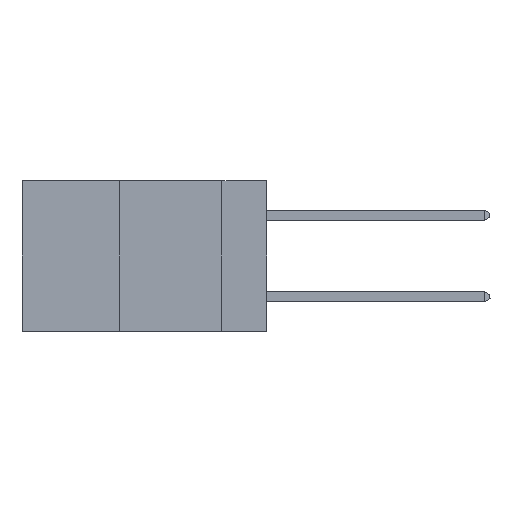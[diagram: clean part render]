
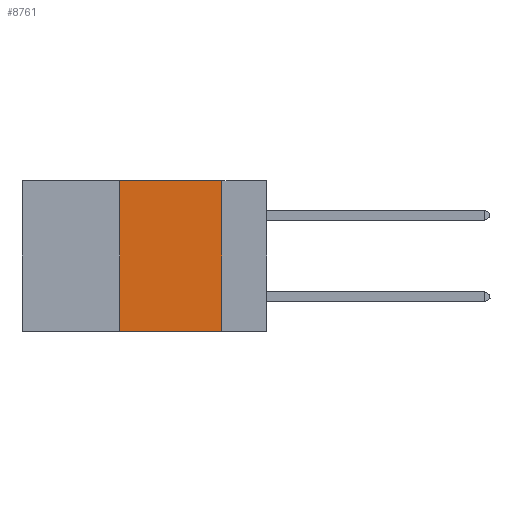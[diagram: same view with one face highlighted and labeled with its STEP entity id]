
A CAD part, left-side view. The second image highlights one B-rep face of the part: STEP entity #8761.
In plain terms, the highlighted planar face has unit normal (-1, 0, 0).
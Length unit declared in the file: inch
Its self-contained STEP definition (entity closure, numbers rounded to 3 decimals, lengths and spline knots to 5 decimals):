
#80 = LINE ( 'NONE', #5714, #9266 ) ;
#611 = DIRECTION ( 'NONE',  ( 0., 0., 1. ) ) ;
#1285 = EDGE_CURVE ( 'NONE', #9797, #2730, #80, .T. ) ;
#1292 = EDGE_CURVE ( 'NONE', #9797, #6318, #3697, .T. ) ;
#1509 = DIRECTION ( 'NONE',  ( 1., 0., 0. ) ) ;
#1845 = ORIENTED_EDGE ( 'NONE', *, *, #2456, .F. ) ;
#1931 = CARTESIAN_POINT ( 'NONE',  ( 0., 0.11, -0.37 ) ) ;
#2225 = FACE_OUTER_BOUND ( 'NONE', #6689, .T. ) ;
#2456 = EDGE_CURVE ( 'NONE', #7040, #6318, #9133, .T. ) ;
#2730 = VERTEX_POINT ( 'NONE', #5146 ) ;
#3697 = LINE ( 'NONE', #6640, #4223 ) ;
#3983 = PLANE ( 'NONE',  #10372 ) ;
#4223 = VECTOR ( 'NONE', #7470, 39.37008 ) ;
#4244 = DIRECTION ( 'NONE',  ( 0., -1., 0. ) ) ;
#4284 = CARTESIAN_POINT ( 'NONE',  ( 0., 0.6, 0. ) ) ;
#4816 = ORIENTED_EDGE ( 'NONE', *, *, #8302, .F. ) ;
#5146 = CARTESIAN_POINT ( 'NONE',  ( 0., 0.36, 0. ) ) ;
#5529 = ORIENTED_EDGE ( 'NONE', *, *, #1292, .T. ) ;
#5714 = CARTESIAN_POINT ( 'NONE',  ( 0., 0.36, 0. ) ) ;
#5935 = DIRECTION ( 'NONE',  ( 0., 0., -1. ) ) ;
#6318 = VERTEX_POINT ( 'NONE', #1931 ) ;
#6640 = CARTESIAN_POINT ( 'NONE',  ( 0., 0.6, -0.37 ) ) ;
#6689 = EDGE_LOOP ( 'NONE', ( #1845, #4816, #7768, #5529 ) ) ;
#6808 = CARTESIAN_POINT ( 'NONE',  ( 0., 0.11, 0. ) ) ;
#7040 = VERTEX_POINT ( 'NONE', #8753 ) ;
#7470 = DIRECTION ( 'NONE',  ( 0., -1., 0. ) ) ;
#7768 = ORIENTED_EDGE ( 'NONE', *, *, #1285, .F. ) ;
#8302 = EDGE_CURVE ( 'NONE', #2730, #7040, #8366, .T. ) ;
#8317 = DIRECTION ( 'NONE',  ( 0., 0., -1. ) ) ;
#8366 = LINE ( 'NONE', #4284, #10728 ) ;
#8753 = CARTESIAN_POINT ( 'NONE',  ( 0., 0.11, 0. ) ) ;
#8761 = ADVANCED_FACE ( 'NONE', ( #2225 ), #3983, .F. ) ;
#9133 = LINE ( 'NONE', #6808, #10577 ) ;
#9266 = VECTOR ( 'NONE', #611, 39.37008 ) ;
#9797 = VERTEX_POINT ( 'NONE', #10012 ) ;
#10012 = CARTESIAN_POINT ( 'NONE',  ( 0., 0.36, -0.37 ) ) ;
#10372 = AXIS2_PLACEMENT_3D ( 'NONE', #10783, #1509, #8317 ) ;
#10577 = VECTOR ( 'NONE', #5935, 39.37008 ) ;
#10728 = VECTOR ( 'NONE', #4244, 39.37008 ) ;
#10783 = CARTESIAN_POINT ( 'NONE',  ( 0., 0.6, 0. ) ) ;
